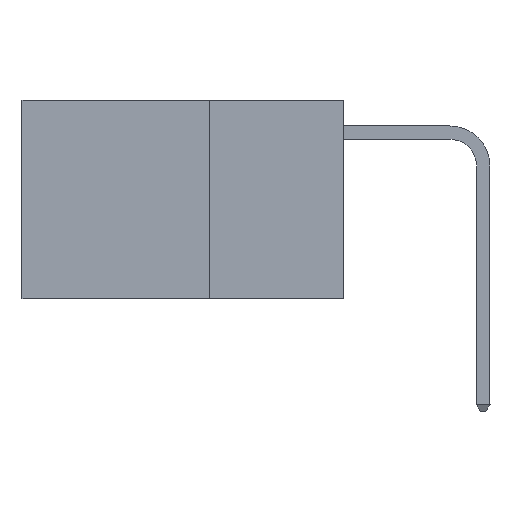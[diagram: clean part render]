
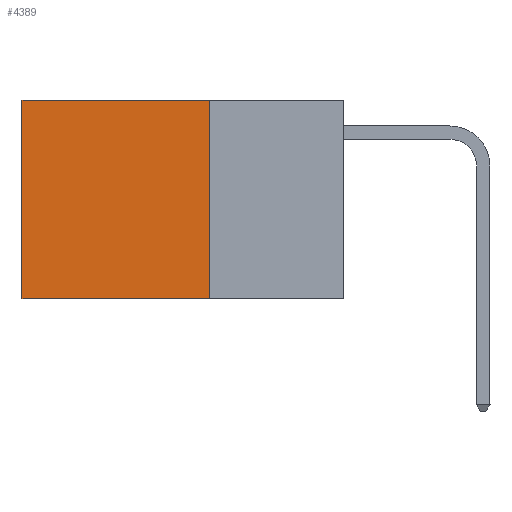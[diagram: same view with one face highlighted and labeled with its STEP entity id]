
A CAD part, left-side view. The second image highlights one B-rep face of the part: STEP entity #4389.
In plain terms, the highlighted planar face has unit normal (-1, 0, 0).
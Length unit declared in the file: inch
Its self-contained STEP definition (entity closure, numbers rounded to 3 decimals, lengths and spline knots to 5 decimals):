
#152 = DIRECTION ( 'NONE',  ( 0., 0., -1. ) ) ;
#528 = CARTESIAN_POINT ( 'NONE',  ( 0.2625, 0.25, -0.37 ) ) ;
#883 = DIRECTION ( 'NONE',  ( 0., 0., -1. ) ) ;
#1085 = CARTESIAN_POINT ( 'NONE',  ( 0.2625, 0.25, 0. ) ) ;
#1156 = PLANE ( 'NONE',  #13894 ) ;
#1552 = EDGE_CURVE ( 'NONE', #12376, #12000, #2324, .T. ) ;
#1882 = CARTESIAN_POINT ( 'NONE',  ( 0.2625, 0.25, 0. ) ) ;
#2009 = CARTESIAN_POINT ( 'NONE',  ( 0.2625, 0.6, -0.37 ) ) ;
#2187 = CARTESIAN_POINT ( 'NONE',  ( 0.2625, 0.25, -0.37 ) ) ;
#2324 = LINE ( 'NONE', #2187, #11838 ) ;
#2510 = CARTESIAN_POINT ( 'NONE',  ( 0.2625, 0.25, 0. ) ) ;
#3064 = VERTEX_POINT ( 'NONE', #1882 ) ;
#3378 = CARTESIAN_POINT ( 'NONE',  ( 0.2625, 0.25, 0. ) ) ;
#3750 = LINE ( 'NONE', #2510, #9639 ) ;
#4197 = CARTESIAN_POINT ( 'NONE',  ( 0.2625, 0.6, 0. ) ) ;
#4389 = ADVANCED_FACE ( 'NONE', ( #8875 ), #1156, .F. ) ;
#4770 = DIRECTION ( 'NONE',  ( 0., 0., -1. ) ) ;
#5288 = LINE ( 'NONE', #4197, #13269 ) ;
#5390 = VERTEX_POINT ( 'NONE', #5787 ) ;
#5548 = DIRECTION ( 'NONE',  ( 0., 1., 0. ) ) ;
#5787 = CARTESIAN_POINT ( 'NONE',  ( 0.2625, 0.6, 0. ) ) ;
#6267 = EDGE_CURVE ( 'NONE', #3064, #5390, #13509, .T. ) ;
#6392 = ORIENTED_EDGE ( 'NONE', *, *, #10581, .F. ) ;
#6729 = DIRECTION ( 'NONE',  ( 0., 1., 0. ) ) ;
#7088 = EDGE_CURVE ( 'NONE', #5390, #12000, #5288, .T. ) ;
#7698 = DIRECTION ( 'NONE',  ( 1., 0., 0. ) ) ;
#7952 = ORIENTED_EDGE ( 'NONE', *, *, #1552, .F. ) ;
#8806 = EDGE_LOOP ( 'NONE', ( #13437, #7952, #6392, #9683 ) ) ;
#8875 = FACE_OUTER_BOUND ( 'NONE', #8806, .T. ) ;
#9639 = VECTOR ( 'NONE', #4770, 39.37008 ) ;
#9683 = ORIENTED_EDGE ( 'NONE', *, *, #6267, .T. ) ;
#10581 = EDGE_CURVE ( 'NONE', #3064, #12376, #3750, .T. ) ;
#11838 = VECTOR ( 'NONE', #6729, 39.37008 ) ;
#12000 = VERTEX_POINT ( 'NONE', #2009 ) ;
#12376 = VERTEX_POINT ( 'NONE', #528 ) ;
#13250 = VECTOR ( 'NONE', #5548, 39.37008 ) ;
#13269 = VECTOR ( 'NONE', #883, 39.37008 ) ;
#13437 = ORIENTED_EDGE ( 'NONE', *, *, #7088, .T. ) ;
#13509 = LINE ( 'NONE', #1085, #13250 ) ;
#13894 = AXIS2_PLACEMENT_3D ( 'NONE', #3378, #7698, #152 ) ;
